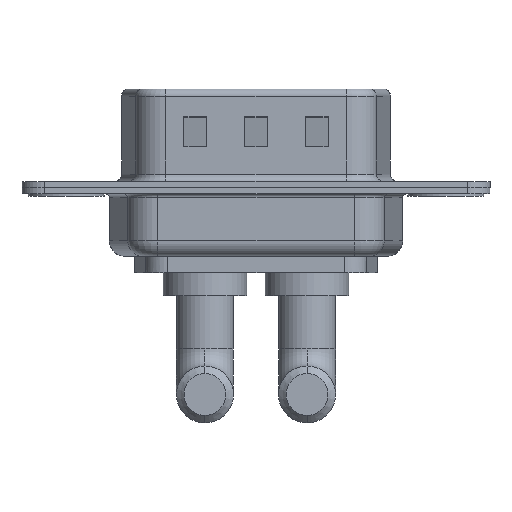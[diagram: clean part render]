
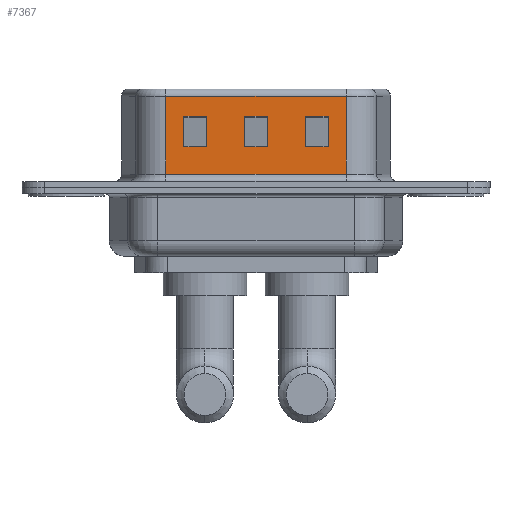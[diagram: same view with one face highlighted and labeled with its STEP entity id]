
A CAD part, front view. The second image highlights one B-rep face of the part: STEP entity #7367.
In plain terms, the highlighted planar face has unit normal (0, -1, 0).
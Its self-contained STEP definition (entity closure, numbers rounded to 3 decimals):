
#30 = ORIENTED_EDGE ( 'NONE', *, *, #780, .T. ) ;
#80 = CARTESIAN_POINT ( 'NONE',  ( 6.549, -4.55, 0.9 ) ) ;
#181 = CARTESIAN_POINT ( 'NONE',  ( 22.451, -4.55, 2.705 ) ) ;
#251 = FACE_BOUND ( 'NONE', #9664, .T. ) ;
#342 = VERTEX_POINT ( 'NONE', #2015 ) ;
#569 = CARTESIAN_POINT ( 'NONE',  ( 9.25, -4.55, 2.705 ) ) ;
#583 = DIRECTION ( 'NONE',  ( 0., 0., -1. ) ) ;
#597 = VECTOR ( 'NONE', #5186, 1000. ) ;
#604 = DIRECTION ( 'NONE',  ( 0., 0., -1. ) ) ;
#651 = CARTESIAN_POINT ( 'NONE',  ( 17.25, -4.55, 4.705 ) ) ;
#727 = VERTEX_POINT ( 'NONE', #9612 ) ;
#754 = EDGE_CURVE ( 'NONE', #1933, #4683, #6695, .T. ) ;
#780 = EDGE_CURVE ( 'NONE', #5630, #1933, #4856, .T. ) ;
#874 = VERTEX_POINT ( 'NONE', #80 ) ;
#1038 = ORIENTED_EDGE ( 'NONE', *, *, #2588, .T. ) ;
#1132 = CARTESIAN_POINT ( 'NONE',  ( 18.451, -4.55, 6.52 ) ) ;
#1144 = VECTOR ( 'NONE', #583, 1000. ) ;
#1165 = VECTOR ( 'NONE', #4677, 1000. ) ;
#1186 = CARTESIAN_POINT ( 'NONE',  ( 7.75, -4.55, 4.705 ) ) ;
#1246 = EDGE_CURVE ( 'NONE', #9688, #1511, #4832, .T. ) ;
#1396 = DIRECTION ( 'NONE',  ( -1., 0., 0. ) ) ;
#1511 = VERTEX_POINT ( 'NONE', #9372 ) ;
#1516 = EDGE_CURVE ( 'NONE', #727, #874, #3555, .T. ) ;
#1529 = CARTESIAN_POINT ( 'NONE',  ( 11.75, -4.55, 6.52 ) ) ;
#1590 = VECTOR ( 'NONE', #2808, 1000. ) ;
#1601 = LINE ( 'NONE', #1676, #6736 ) ;
#1669 = LINE ( 'NONE', #1529, #12150 ) ;
#1676 = CARTESIAN_POINT ( 'NONE',  ( 7.75, -4.55, 6.52 ) ) ;
#1816 = CARTESIAN_POINT ( 'NONE',  ( 7.75, -4.55, 2.705 ) ) ;
#1933 = VERTEX_POINT ( 'NONE', #651 ) ;
#2015 = CARTESIAN_POINT ( 'NONE',  ( 13.25, -4.55, 4.705 ) ) ;
#2034 = EDGE_LOOP ( 'NONE', ( #3187, #5953, #4003, #3069 ) ) ;
#2061 = EDGE_CURVE ( 'NONE', #342, #4109, #12275, .T. ) ;
#2075 = CARTESIAN_POINT ( 'NONE',  ( 11.75, -4.55, 2.705 ) ) ;
#2104 = EDGE_CURVE ( 'NONE', #6307, #7009, #7519, .T. ) ;
#2171 = FACE_BOUND ( 'NONE', #3131, .T. ) ;
#2482 = VECTOR ( 'NONE', #3199, 1000. ) ;
#2588 = EDGE_CURVE ( 'NONE', #4109, #2794, #7525, .T. ) ;
#2737 = LINE ( 'NONE', #3868, #8374 ) ;
#2794 = VERTEX_POINT ( 'NONE', #2075 ) ;
#2808 = DIRECTION ( 'NONE',  ( 0., 0., -1. ) ) ;
#2829 = EDGE_CURVE ( 'NONE', #10057, #6307, #10641, .T. ) ;
#3016 = VERTEX_POINT ( 'NONE', #12567 ) ;
#3069 = ORIENTED_EDGE ( 'NONE', *, *, #10424, .T. ) ;
#3071 = CARTESIAN_POINT ( 'NONE',  ( 18.451, -4.55, 6.52 ) ) ;
#3131 = EDGE_LOOP ( 'NONE', ( #8946, #6912, #8897, #6372 ) ) ;
#3187 = ORIENTED_EDGE ( 'NONE', *, *, #1246, .F. ) ;
#3199 = DIRECTION ( 'NONE',  ( 1., 0., 0. ) ) ;
#3441 = VERTEX_POINT ( 'NONE', #8694 ) ;
#3543 = CARTESIAN_POINT ( 'NONE',  ( 18.451, -4.55, 2.705 ) ) ;
#3555 = LINE ( 'NONE', #11344, #8499 ) ;
#3868 = CARTESIAN_POINT ( 'NONE',  ( 15.75, -4.55, 6.52 ) ) ;
#3908 = CARTESIAN_POINT ( 'NONE',  ( 17.25, -4.55, 6.52 ) ) ;
#3916 = DIRECTION ( 'NONE',  ( 1., 0., 0. ) ) ;
#4003 = ORIENTED_EDGE ( 'NONE', *, *, #1516, .T. ) ;
#4069 = DIRECTION ( 'NONE',  ( -1., 0., 0. ) ) ;
#4109 = VERTEX_POINT ( 'NONE', #9681 ) ;
#4189 = EDGE_CURVE ( 'NONE', #3441, #342, #7065, .T. ) ;
#4383 = EDGE_CURVE ( 'NONE', #3016, #5630, #2737, .T. ) ;
#4409 = CARTESIAN_POINT ( 'NONE',  ( 13.25, -4.55, 6.52 ) ) ;
#4596 = DIRECTION ( 'NONE',  ( 0., 0., 1. ) ) ;
#4642 = ORIENTED_EDGE ( 'NONE', *, *, #4383, .T. ) ;
#4665 = DIRECTION ( 'NONE',  ( 1., 0., 0. ) ) ;
#4677 = DIRECTION ( 'NONE',  ( -1., 0., 0. ) ) ;
#4683 = VERTEX_POINT ( 'NONE', #8171 ) ;
#4749 = ORIENTED_EDGE ( 'NONE', *, *, #754, .T. ) ;
#4768 = ORIENTED_EDGE ( 'NONE', *, *, #5502, .T. ) ;
#4796 = CARTESIAN_POINT ( 'NONE',  ( 22.451, -4.55, 4.705 ) ) ;
#4832 = LINE ( 'NONE', #1132, #1590 ) ;
#4856 = LINE ( 'NONE', #4796, #8679 ) ;
#5084 = DIRECTION ( 'NONE',  ( -1., 0., 0. ) ) ;
#5186 = DIRECTION ( 'NONE',  ( -1., 0., 0. ) ) ;
#5398 = DIRECTION ( 'NONE',  ( 0., 0., 1. ) ) ;
#5502 = EDGE_CURVE ( 'NONE', #4683, #3016, #8840, .T. ) ;
#5614 = CARTESIAN_POINT ( 'NONE',  ( 9.25, -4.55, 6.52 ) ) ;
#5630 = VERTEX_POINT ( 'NONE', #10469 ) ;
#5717 = VECTOR ( 'NONE', #1396, 1000. ) ;
#5754 = VECTOR ( 'NONE', #3916, 1000. ) ;
#5953 = ORIENTED_EDGE ( 'NONE', *, *, #10105, .T. ) ;
#5962 = CARTESIAN_POINT ( 'NONE',  ( 18.451, -4.55, 6.02 ) ) ;
#6270 = CARTESIAN_POINT ( 'NONE',  ( 9.25, -4.55, 4.705 ) ) ;
#6307 = VERTEX_POINT ( 'NONE', #6270 ) ;
#6372 = ORIENTED_EDGE ( 'NONE', *, *, #2829, .T. ) ;
#6653 = LINE ( 'NONE', #6783, #6914 ) ;
#6695 = LINE ( 'NONE', #3908, #7037 ) ;
#6736 = VECTOR ( 'NONE', #4596, 1000. ) ;
#6783 = CARTESIAN_POINT ( 'NONE',  ( 18.451, -4.55, 0.9 ) ) ;
#6912 = ORIENTED_EDGE ( 'NONE', *, *, #7406, .T. ) ;
#6914 = VECTOR ( 'NONE', #9636, 1000. ) ;
#6932 = DIRECTION ( 'NONE',  ( 0., 1., 0. ) ) ;
#6935 = AXIS2_PLACEMENT_3D ( 'NONE', #3071, #6932, #5084 ) ;
#7009 = VERTEX_POINT ( 'NONE', #569 ) ;
#7037 = VECTOR ( 'NONE', #10444, 1000. ) ;
#7065 = LINE ( 'NONE', #7253, #2482 ) ;
#7253 = CARTESIAN_POINT ( 'NONE',  ( 18.451, -4.55, 4.705 ) ) ;
#7367 = ADVANCED_FACE ( 'NONE', ( #2171, #251, #7887, #9908 ), #11757, .F. ) ;
#7406 = EDGE_CURVE ( 'NONE', #7009, #8016, #9204, .T. ) ;
#7519 = LINE ( 'NONE', #5614, #12499 ) ;
#7525 = LINE ( 'NONE', #3543, #1165 ) ;
#7620 = ORIENTED_EDGE ( 'NONE', *, *, #2061, .T. ) ;
#7887 = FACE_BOUND ( 'NONE', #7908, .T. ) ;
#7908 = EDGE_LOOP ( 'NONE', ( #10739, #7620, #1038, #8727 ) ) ;
#8016 = VERTEX_POINT ( 'NONE', #1816 ) ;
#8107 = LINE ( 'NONE', #5962, #597 ) ;
#8171 = CARTESIAN_POINT ( 'NONE',  ( 17.25, -4.55, 2.705 ) ) ;
#8374 = VECTOR ( 'NONE', #10406, 1000. ) ;
#8499 = VECTOR ( 'NONE', #604, 1000. ) ;
#8679 = VECTOR ( 'NONE', #4665, 1000. ) ;
#8694 = CARTESIAN_POINT ( 'NONE',  ( 11.75, -4.55, 4.705 ) ) ;
#8727 = ORIENTED_EDGE ( 'NONE', *, *, #9956, .T. ) ;
#8738 = CARTESIAN_POINT ( 'NONE',  ( 14.451, -4.55, 4.705 ) ) ;
#8840 = LINE ( 'NONE', #181, #12136 ) ;
#8897 = ORIENTED_EDGE ( 'NONE', *, *, #11252, .T. ) ;
#8946 = ORIENTED_EDGE ( 'NONE', *, *, #2104, .T. ) ;
#9204 = LINE ( 'NONE', #12182, #5717 ) ;
#9372 = CARTESIAN_POINT ( 'NONE',  ( 18.451, -4.55, 0.9 ) ) ;
#9612 = CARTESIAN_POINT ( 'NONE',  ( 6.549, -4.55, 6.02 ) ) ;
#9636 = DIRECTION ( 'NONE',  ( 1., 0., 0. ) ) ;
#9664 = EDGE_LOOP ( 'NONE', ( #4749, #4768, #4642, #30 ) ) ;
#9668 = CARTESIAN_POINT ( 'NONE',  ( 18.451, -4.55, 6.02 ) ) ;
#9681 = CARTESIAN_POINT ( 'NONE',  ( 13.25, -4.55, 2.705 ) ) ;
#9688 = VERTEX_POINT ( 'NONE', #9668 ) ;
#9908 = FACE_OUTER_BOUND ( 'NONE', #2034, .T. ) ;
#9956 = EDGE_CURVE ( 'NONE', #2794, #3441, #1669, .T. ) ;
#10057 = VERTEX_POINT ( 'NONE', #1186 ) ;
#10105 = EDGE_CURVE ( 'NONE', #9688, #727, #8107, .T. ) ;
#10406 = DIRECTION ( 'NONE',  ( 0., 0., 1. ) ) ;
#10424 = EDGE_CURVE ( 'NONE', #874, #1511, #6653, .T. ) ;
#10444 = DIRECTION ( 'NONE',  ( 0., 0., -1. ) ) ;
#10469 = CARTESIAN_POINT ( 'NONE',  ( 15.75, -4.55, 4.705 ) ) ;
#10641 = LINE ( 'NONE', #8738, #5754 ) ;
#10739 = ORIENTED_EDGE ( 'NONE', *, *, #4189, .T. ) ;
#11252 = EDGE_CURVE ( 'NONE', #8016, #10057, #1601, .T. ) ;
#11344 = CARTESIAN_POINT ( 'NONE',  ( 6.549, -4.55, 6.52 ) ) ;
#11392 = DIRECTION ( 'NONE',  ( 0., 0., -1. ) ) ;
#11757 = PLANE ( 'NONE',  #6935 ) ;
#12136 = VECTOR ( 'NONE', #4069, 1000. ) ;
#12150 = VECTOR ( 'NONE', #5398, 1000. ) ;
#12182 = CARTESIAN_POINT ( 'NONE',  ( 14.451, -4.55, 2.705 ) ) ;
#12275 = LINE ( 'NONE', #4409, #1144 ) ;
#12499 = VECTOR ( 'NONE', #11392, 1000. ) ;
#12567 = CARTESIAN_POINT ( 'NONE',  ( 15.75, -4.55, 2.705 ) ) ;
